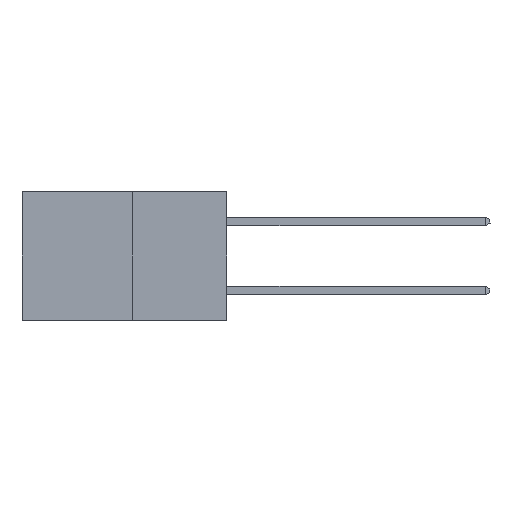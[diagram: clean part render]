
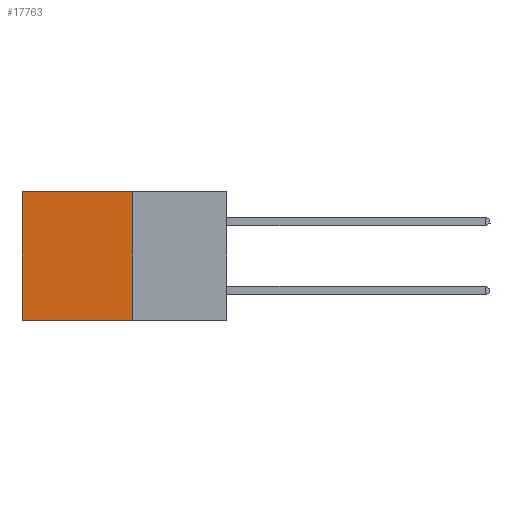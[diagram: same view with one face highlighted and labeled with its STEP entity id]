
A CAD part, left-side view. The second image highlights one B-rep face of the part: STEP entity #17763.
In plain terms, the highlighted planar face has unit normal (-1, 0, 0).
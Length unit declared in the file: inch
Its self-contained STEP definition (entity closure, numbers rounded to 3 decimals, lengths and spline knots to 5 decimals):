
#224 = ORIENTED_EDGE ( 'NONE', *, *, #12884, .F. ) ;
#1028 = DIRECTION ( 'NONE',  ( 0., 0., -1. ) ) ;
#1248 = LINE ( 'NONE', #11085, #12264 ) ;
#1275 = CARTESIAN_POINT ( 'NONE',  ( 0.277, 0.27, -0.37 ) ) ;
#1849 = DIRECTION ( 'NONE',  ( 0., 1., 0. ) ) ;
#2010 = DIRECTION ( 'NONE',  ( 0., 0., -1. ) ) ;
#2529 = ORIENTED_EDGE ( 'NONE', *, *, #11142, .T. ) ;
#2614 = VERTEX_POINT ( 'NONE', #8406 ) ;
#4009 = VECTOR ( 'NONE', #2010, 39.37008 ) ;
#4162 = PLANE ( 'NONE',  #11084 ) ;
#4988 = EDGE_LOOP ( 'NONE', ( #10098, #224, #15375, #2529 ) ) ;
#5355 = CARTESIAN_POINT ( 'NONE',  ( 0.277, 0.27, -0.37 ) ) ;
#5568 = DIRECTION ( 'NONE',  ( 0., 0., -1. ) ) ;
#5794 = CARTESIAN_POINT ( 'NONE',  ( 0.277, 0.27, -0.37 ) ) ;
#6085 = LINE ( 'NONE', #10449, #9022 ) ;
#7377 = EDGE_CURVE ( 'NONE', #8301, #17612, #8228, .T. ) ;
#8228 = LINE ( 'NONE', #12081, #4009 ) ;
#8264 = LINE ( 'NONE', #5355, #15552 ) ;
#8301 = VERTEX_POINT ( 'NONE', #18582 ) ;
#8406 = CARTESIAN_POINT ( 'NONE',  ( 0.277, 0.27, 0. ) ) ;
#8866 = EDGE_CURVE ( 'NONE', #2614, #10368, #1248, .T. ) ;
#9022 = VECTOR ( 'NONE', #1849, 39.37008 ) ;
#10098 = ORIENTED_EDGE ( 'NONE', *, *, #7377, .T. ) ;
#10368 = VERTEX_POINT ( 'NONE', #5794 ) ;
#10449 = CARTESIAN_POINT ( 'NONE',  ( 0.277, 0.27, 0. ) ) ;
#11084 = AXIS2_PLACEMENT_3D ( 'NONE', #1275, #14235, #5568 ) ;
#11085 = CARTESIAN_POINT ( 'NONE',  ( 0.277, 0.27, -0.37 ) ) ;
#11142 = EDGE_CURVE ( 'NONE', #2614, #8301, #6085, .T. ) ;
#12081 = CARTESIAN_POINT ( 'NONE',  ( 0.277, 0.59, -0.37 ) ) ;
#12264 = VECTOR ( 'NONE', #1028, 39.37008 ) ;
#12611 = DIRECTION ( 'NONE',  ( 0., 1., 0. ) ) ;
#12884 = EDGE_CURVE ( 'NONE', #10368, #17612, #8264, .T. ) ;
#14235 = DIRECTION ( 'NONE',  ( 1., 0., 0. ) ) ;
#15375 = ORIENTED_EDGE ( 'NONE', *, *, #8866, .F. ) ;
#15552 = VECTOR ( 'NONE', #12611, 39.37008 ) ;
#16774 = FACE_OUTER_BOUND ( 'NONE', #4988, .T. ) ;
#16854 = CARTESIAN_POINT ( 'NONE',  ( 0.277, 0.59, -0.37 ) ) ;
#17612 = VERTEX_POINT ( 'NONE', #16854 ) ;
#17763 = ADVANCED_FACE ( 'NONE', ( #16774 ), #4162, .F. ) ;
#18582 = CARTESIAN_POINT ( 'NONE',  ( 0.277, 0.59, 0. ) ) ;
